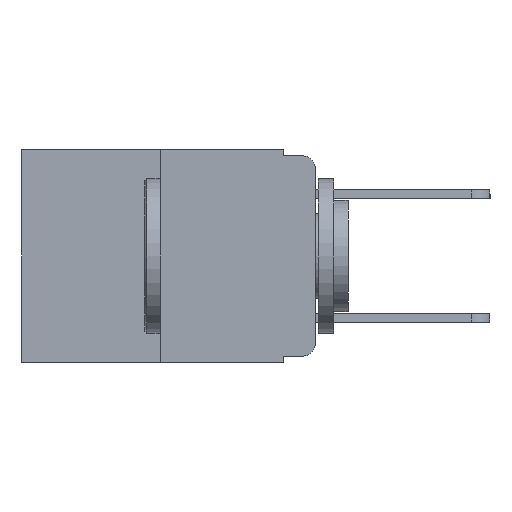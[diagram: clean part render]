
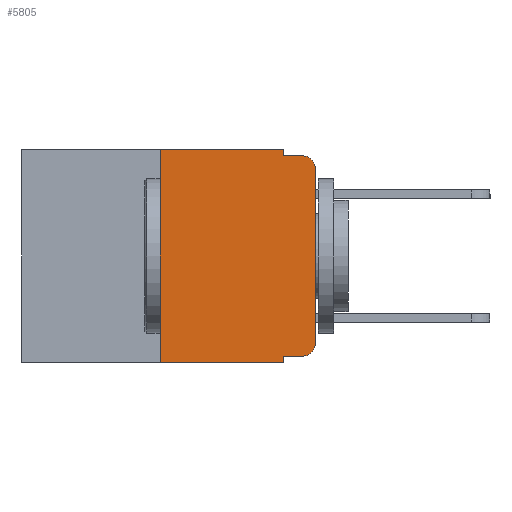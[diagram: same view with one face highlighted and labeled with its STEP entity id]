
A CAD part, left-side view. The second image highlights one B-rep face of the part: STEP entity #5805.
In plain terms, the highlighted planar face has unit normal (-1, 0, 0).
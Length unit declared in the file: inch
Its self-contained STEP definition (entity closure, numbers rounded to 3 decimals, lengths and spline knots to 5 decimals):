
#27 = ORIENTED_EDGE ( 'NONE', *, *, #8594, .T. ) ;
#115 = CARTESIAN_POINT ( 'NONE',  ( 0., 0.051, -0.343 ) ) ;
#451 = EDGE_LOOP ( 'NONE', ( #2738, #7040, #11703, #4194, #4437, #3678, #5434, #6412, #4814, #27 ) ) ;
#453 = VERTEX_POINT ( 'NONE', #2895 ) ;
#486 = EDGE_CURVE ( 'NONE', #2441, #3170, #8546, .T. ) ;
#613 = VERTEX_POINT ( 'NONE', #9541 ) ;
#785 = CARTESIAN_POINT ( 'NONE',  ( 0., 0.051, 0. ) ) ;
#828 = VECTOR ( 'NONE', #7895, 39.37008 ) ;
#900 = DIRECTION ( 'NONE',  ( 0., 0., -1. ) ) ;
#1003 = EDGE_CURVE ( 'NONE', #613, #3170, #6676, .T. ) ;
#1791 = VECTOR ( 'NONE', #900, 39.37008 ) ;
#2065 = EDGE_CURVE ( 'NONE', #7920, #613, #5402, .T. ) ;
#2211 = VERTEX_POINT ( 'NONE', #6439 ) ;
#2246 = DIRECTION ( 'NONE',  ( 0., 0., 1. ) ) ;
#2376 = VERTEX_POINT ( 'NONE', #115 ) ;
#2441 = VERTEX_POINT ( 'NONE', #2769 ) ;
#2626 = VERTEX_POINT ( 'NONE', #9109 ) ;
#2649 = VERTEX_POINT ( 'NONE', #6668 ) ;
#2673 = DIRECTION ( 'NONE',  ( 1., 0., 0. ) ) ;
#2738 = ORIENTED_EDGE ( 'NONE', *, *, #2065, .T. ) ;
#2769 = CARTESIAN_POINT ( 'NONE',  ( 0., 0.051, -0.01 ) ) ;
#2895 = CARTESIAN_POINT ( 'NONE',  ( 0., 0.051, 0. ) ) ;
#3080 = PLANE ( 'NONE',  #10217 ) ;
#3170 = VERTEX_POINT ( 'NONE', #9951 ) ;
#3325 = VECTOR ( 'NONE', #4921, 39.37008 ) ;
#3459 = CARTESIAN_POINT ( 'NONE',  ( 0., 0.473, 0. ) ) ;
#3678 = ORIENTED_EDGE ( 'NONE', *, *, #11202, .F. ) ;
#3714 = LINE ( 'NONE', #4950, #3325 ) ;
#4194 = ORIENTED_EDGE ( 'NONE', *, *, #6878, .F. ) ;
#4230 = LINE ( 'NONE', #5587, #10940 ) ;
#4409 = DIRECTION ( 'NONE',  ( 0., -1., 0. ) ) ;
#4429 = LINE ( 'NONE', #10541, #828 ) ;
#4437 = ORIENTED_EDGE ( 'NONE', *, *, #9201, .F. ) ;
#4814 = ORIENTED_EDGE ( 'NONE', *, *, #8731, .T. ) ;
#4921 = DIRECTION ( 'NONE',  ( 0., -1., 0. ) ) ;
#4931 = LINE ( 'NONE', #785, #1791 ) ;
#4950 = CARTESIAN_POINT ( 'NONE',  ( 0., 0.051, -0.333 ) ) ;
#5376 = DIRECTION ( 'NONE',  ( 0., -1., 0. ) ) ;
#5402 = LINE ( 'NONE', #9302, #12102 ) ;
#5434 = ORIENTED_EDGE ( 'NONE', *, *, #6109, .T. ) ;
#5587 = CARTESIAN_POINT ( 'NONE',  ( 0., 0.473, 0. ) ) ;
#5613 = VECTOR ( 'NONE', #12500, 39.37008 ) ;
#5805 = ADVANCED_FACE ( 'NONE', ( #6889 ), #3080, .F. ) ;
#5912 = LINE ( 'NONE', #10159, #5613 ) ;
#6109 = EDGE_CURVE ( 'NONE', #2211, #2376, #5912, .T. ) ;
#6148 = VERTEX_POINT ( 'NONE', #11583 ) ;
#6235 = CARTESIAN_POINT ( 'NONE',  ( 0., 0.051, 0. ) ) ;
#6238 = DIRECTION ( 'NONE',  ( 0., 0., -1. ) ) ;
#6412 = ORIENTED_EDGE ( 'NONE', *, *, #8101, .F. ) ;
#6439 = CARTESIAN_POINT ( 'NONE',  ( 0., 0.25, -0.343 ) ) ;
#6668 = CARTESIAN_POINT ( 'NONE',  ( 0., 0.25, 0. ) ) ;
#6676 = CIRCLE ( 'NONE', #7188, 0.02 ) ;
#6875 = DIRECTION ( 'NONE',  ( 0., 0., -1. ) ) ;
#6878 = EDGE_CURVE ( 'NONE', #453, #2441, #7741, .T. ) ;
#6888 = DIRECTION ( 'NONE',  ( -1., 0., 0. ) ) ;
#6889 = FACE_OUTER_BOUND ( 'NONE', #451, .T. ) ;
#6920 = CARTESIAN_POINT ( 'NONE',  ( 0., 0.02, -0.313 ) ) ;
#7040 = ORIENTED_EDGE ( 'NONE', *, *, #1003, .T. ) ;
#7089 = AXIS2_PLACEMENT_3D ( 'NONE', #6920, #6888, #6875 ) ;
#7188 = AXIS2_PLACEMENT_3D ( 'NONE', #9809, #9827, #11417 ) ;
#7741 = LINE ( 'NONE', #6235, #12515 ) ;
#7755 = CARTESIAN_POINT ( 'NONE',  ( 0., 0., -0.313 ) ) ;
#7895 = DIRECTION ( 'NONE',  ( 0., 0., 1. ) ) ;
#7920 = VERTEX_POINT ( 'NONE', #7755 ) ;
#8101 = EDGE_CURVE ( 'NONE', #6148, #2376, #4931, .T. ) ;
#8546 = LINE ( 'NONE', #9946, #12477 ) ;
#8594 = EDGE_CURVE ( 'NONE', #2626, #7920, #12581, .T. ) ;
#8731 = EDGE_CURVE ( 'NONE', #6148, #2626, #3714, .T. ) ;
#9109 = CARTESIAN_POINT ( 'NONE',  ( 0., 0.02, -0.333 ) ) ;
#9201 = EDGE_CURVE ( 'NONE', #2649, #453, #4230, .T. ) ;
#9302 = CARTESIAN_POINT ( 'NONE',  ( 0., 0., 0. ) ) ;
#9377 = DIRECTION ( 'NONE',  ( 0., 0., -1. ) ) ;
#9541 = CARTESIAN_POINT ( 'NONE',  ( 0., 0., -0.03 ) ) ;
#9809 = CARTESIAN_POINT ( 'NONE',  ( 0., 0.02, -0.03 ) ) ;
#9827 = DIRECTION ( 'NONE',  ( -1., 0., 0. ) ) ;
#9946 = CARTESIAN_POINT ( 'NONE',  ( 0., 0.051, -0.01 ) ) ;
#9951 = CARTESIAN_POINT ( 'NONE',  ( 0., 0.02, -0.01 ) ) ;
#10159 = CARTESIAN_POINT ( 'NONE',  ( 0., 0.473, -0.343 ) ) ;
#10217 = AXIS2_PLACEMENT_3D ( 'NONE', #3459, #2673, #9377 ) ;
#10541 = CARTESIAN_POINT ( 'NONE',  ( 0., 0.25, 0. ) ) ;
#10940 = VECTOR ( 'NONE', #5376, 39.37008 ) ;
#11202 = EDGE_CURVE ( 'NONE', #2211, #2649, #4429, .T. ) ;
#11417 = DIRECTION ( 'NONE',  ( 0., 0., -1. ) ) ;
#11583 = CARTESIAN_POINT ( 'NONE',  ( 0., 0.051, -0.333 ) ) ;
#11703 = ORIENTED_EDGE ( 'NONE', *, *, #486, .F. ) ;
#12102 = VECTOR ( 'NONE', #2246, 39.37008 ) ;
#12477 = VECTOR ( 'NONE', #4409, 39.37008 ) ;
#12500 = DIRECTION ( 'NONE',  ( 0., -1., 0. ) ) ;
#12515 = VECTOR ( 'NONE', #6238, 39.37008 ) ;
#12581 = CIRCLE ( 'NONE', #7089, 0.02 ) ;
